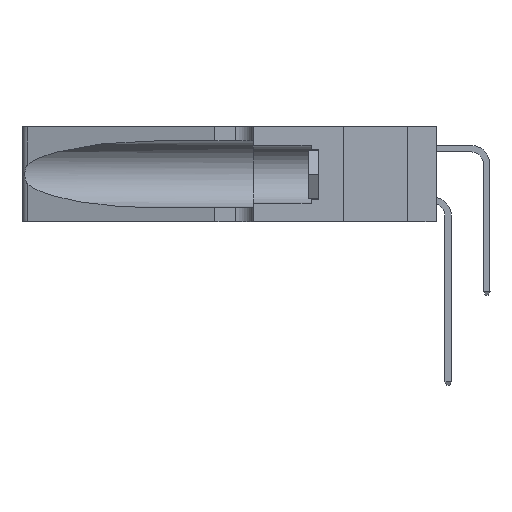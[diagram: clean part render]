
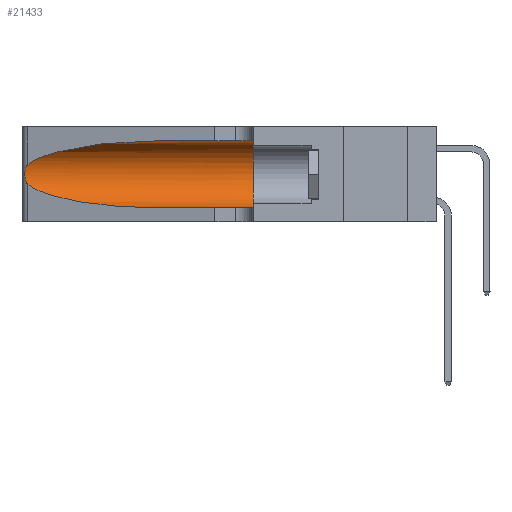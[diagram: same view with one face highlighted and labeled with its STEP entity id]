
A CAD part, left-side view. The second image highlights one B-rep face of the part: STEP entity #21433.
In plain terms, the highlighted cylindrical face has radius 3.308 mm (diameter 6.617 mm), a partial arc.
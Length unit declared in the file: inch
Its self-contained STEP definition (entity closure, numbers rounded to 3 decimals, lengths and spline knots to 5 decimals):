
#247 = CARTESIAN_POINT ( 'NONE',  ( 0.1305, 1.61858, 0.185 ) ) ;
#335 = VECTOR ( 'NONE', #14782, 39.37008 ) ;
#343 =( BOUNDED_CURVE ( )  B_SPLINE_CURVE ( 3, ( #13211, #21269, #7963, #26516 ),
 .UNSPECIFIED., .F., .T. ) 
 B_SPLINE_CURVE_WITH_KNOTS ( ( 4, 4 ),
 ( 1.5708, 2.84003 ),
 .UNSPECIFIED. ) 
 CURVE ( )  GEOMETRIC_REPRESENTATION_ITEM ( )  RATIONAL_B_SPLINE_CURVE ( ( 1., 0.87, 0.87, 1. ) ) 
 REPRESENTATION_ITEM ( '' )  );
#814 = CARTESIAN_POINT ( 'NONE',  ( 0.25487, 1.22718, 0.14631 ) ) ;
#829 = CARTESIAN_POINT ( 'NONE',  ( 0.26075, 1.23896, 0.178 ) ) ;
#1227 = CARTESIAN_POINT ( 'NONE',  ( 0.25487, 1.22718, 0.22369 ) ) ;
#1411 = CIRCLE ( 'NONE', #30948, 0.13025 ) ;
#2063 = EDGE_CURVE ( 'NONE', #14466, #10567, #9121, .T. ) ;
#2746 = EDGE_CURVE ( 'NONE', #10567, #4013, #13102, .T. ) ;
#2951 = DIRECTION ( 'NONE',  ( 0., 0., -1. ) ) ;
#3510 = CARTESIAN_POINT ( 'NONE',  ( 0.25856, 1.23593, 0.16098 ) ) ;
#4013 = VERTEX_POINT ( 'NONE', #25594 ) ;
#4072 = ORIENTED_EDGE ( 'NONE', *, *, #5862, .F. ) ;
#5862 = EDGE_CURVE ( 'NONE', #21548, #28185, #21633, .T. ) ;
#6183 = CARTESIAN_POINT ( 'NONE',  ( 0.25639, 1.23186, 0.15144 ) ) ;
#6963 = CARTESIAN_POINT ( 'NONE',  ( 0.1305, 0.72297, 0.05475 ) ) ;
#7963 = CARTESIAN_POINT ( 'NONE',  ( 0.2373, 1.15595, 0.28018 ) ) ;
#8564 = EDGE_CURVE ( 'NONE', #11134, #14466, #18948, .T. ) ;
#8860 = CARTESIAN_POINT ( 'NONE',  ( 0.25487, 1.22718, 0.14631 ) ) ;
#9121 =( BOUNDED_CURVE ( )  B_SPLINE_CURVE ( 3, ( #27862, #22610, #33010, #11998 ),
 .UNSPECIFIED., .F., .F. ) 
 B_SPLINE_CURVE_WITH_KNOTS ( ( 4, 4 ),
 ( 3.44316, 4.71239 ),
 .UNSPECIFIED. ) 
 CURVE ( )  GEOMETRIC_REPRESENTATION_ITEM ( )  RATIONAL_B_SPLINE_CURVE ( ( 1., 0.87, 0.87, 1. ) ) 
 REPRESENTATION_ITEM ( '' )  );
#10222 = ORIENTED_EDGE ( 'NONE', *, *, #2746, .T. ) ;
#10567 = VERTEX_POINT ( 'NONE', #6963 ) ;
#11134 = VERTEX_POINT ( 'NONE', #1227 ) ;
#11276 = CARTESIAN_POINT ( 'NONE',  ( 0.1305, 0.35, 0.185 ) ) ;
#11300 = CARTESIAN_POINT ( 'NONE',  ( 0.25487, 1.22718, 0.22369 ) ) ;
#11420 = CARTESIAN_POINT ( 'NONE',  ( 0.25639, 1.23184, 0.21858 ) ) ;
#11998 = CARTESIAN_POINT ( 'NONE',  ( 0.1305, 0.72297, 0.05475 ) ) ;
#12345 = EDGE_CURVE ( 'NONE', #28185, #4013, #1411, .T. ) ;
#12847 = FACE_OUTER_BOUND ( 'NONE', #29449, .T. ) ;
#13102 = LINE ( 'NONE', #30572, #27167 ) ;
#13211 = CARTESIAN_POINT ( 'NONE',  ( 0.1305, 0.72297, 0.31525 ) ) ;
#13990 = DIRECTION ( 'NONE',  ( 0., 0., 1. ) ) ;
#14128 = CARTESIAN_POINT ( 'NONE',  ( 0.25854, 1.2359, 0.20912 ) ) ;
#14466 = VERTEX_POINT ( 'NONE', #814 ) ;
#14761 = DIRECTION ( 'NONE',  ( 0., -1., 0. ) ) ;
#14782 = DIRECTION ( 'NONE',  ( 0., -1., 0. ) ) ;
#15667 = EDGE_CURVE ( 'NONE', #21548, #11134, #343, .T. ) ;
#16786 = CARTESIAN_POINT ( 'NONE',  ( 0.26075, 1.23896, 0.19203 ) ) ;
#17394 = CARTESIAN_POINT ( 'NONE',  ( 0.1305, 0.35, 0.31525 ) ) ;
#18948 = B_SPLINE_CURVE_WITH_KNOTS ( 'NONE', 3,
 ( #11300, #24679, #11420, #29934, #14128, #32566, #16786, #829, #19464, #3510, #22161, #6183, #24795, #8860 ),
 .UNSPECIFIED., .F., .F.,
 ( 4, 2, 2, 2, 2, 2, 4 ),
 ( 0., 0.00027, 0.00053, 0.00107, 0.0016, 0.00187, 0.00214 ),
 .UNSPECIFIED. ) ;
#19464 = CARTESIAN_POINT ( 'NONE',  ( 0.26017, 1.23833, 0.17102 ) ) ;
#19622 = ORIENTED_EDGE ( 'NONE', *, *, #15667, .T. ) ;
#21113 = ORIENTED_EDGE ( 'NONE', *, *, #2063, .T. ) ;
#21269 = CARTESIAN_POINT ( 'NONE',  ( 0.18966, 0.96281, 0.31525 ) ) ;
#21433 = ADVANCED_FACE ( 'NONE', ( #12847 ), #33087, .F. ) ;
#21548 = VERTEX_POINT ( 'NONE', #22068 ) ;
#21633 = LINE ( 'NONE', #33212, #335 ) ;
#22068 = CARTESIAN_POINT ( 'NONE',  ( 0.1305, 0.72297, 0.31525 ) ) ;
#22161 = CARTESIAN_POINT ( 'NONE',  ( 0.25789, 1.23486, 0.15765 ) ) ;
#22610 = CARTESIAN_POINT ( 'NONE',  ( 0.2373, 1.15595, 0.08982 ) ) ;
#24679 = CARTESIAN_POINT ( 'NONE',  ( 0.25555, 1.22994, 0.2215 ) ) ;
#24795 = CARTESIAN_POINT ( 'NONE',  ( 0.25555, 1.22993, 0.14849 ) ) ;
#25594 = CARTESIAN_POINT ( 'NONE',  ( 0.1305, 0.35, 0.05475 ) ) ;
#26209 = AXIS2_PLACEMENT_3D ( 'NONE', #247, #26750, #2951 ) ;
#26516 = CARTESIAN_POINT ( 'NONE',  ( 0.25487, 1.22718, 0.22369 ) ) ;
#26750 = DIRECTION ( 'NONE',  ( 0., -1., 0. ) ) ;
#27167 = VECTOR ( 'NONE', #14761, 39.37008 ) ;
#27862 = CARTESIAN_POINT ( 'NONE',  ( 0.25487, 1.22718, 0.14631 ) ) ;
#28185 = VERTEX_POINT ( 'NONE', #17394 ) ;
#29219 = ORIENTED_EDGE ( 'NONE', *, *, #8564, .T. ) ;
#29449 = EDGE_LOOP ( 'NONE', ( #19622, #29219, #21113, #10222, #30907, #4072 ) ) ;
#29791 = DIRECTION ( 'NONE',  ( 0., 1., 0. ) ) ;
#29934 = CARTESIAN_POINT ( 'NONE',  ( 0.25787, 1.23484, 0.2124 ) ) ;
#30572 = CARTESIAN_POINT ( 'NONE',  ( 0.1305, 1.61858, 0.05475 ) ) ;
#30907 = ORIENTED_EDGE ( 'NONE', *, *, #12345, .F. ) ;
#30948 = AXIS2_PLACEMENT_3D ( 'NONE', #11276, #29791, #13990 ) ;
#32566 = CARTESIAN_POINT ( 'NONE',  ( 0.26018, 1.23835, 0.19895 ) ) ;
#33010 = CARTESIAN_POINT ( 'NONE',  ( 0.18966, 0.96281, 0.05475 ) ) ;
#33087 = CYLINDRICAL_SURFACE ( 'NONE', #26209, 0.13025 ) ;
#33212 = CARTESIAN_POINT ( 'NONE',  ( 0.1305, 1.61858, 0.31525 ) ) ;
